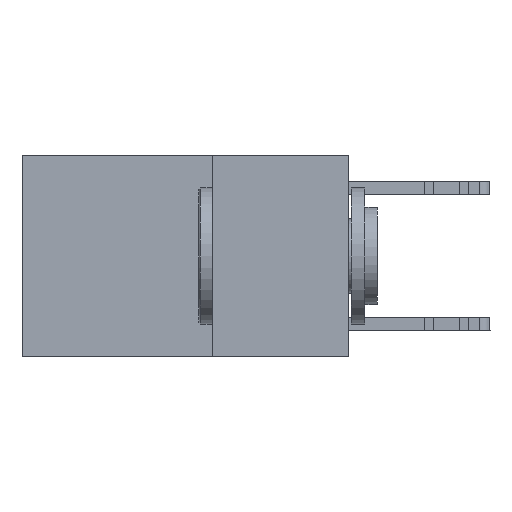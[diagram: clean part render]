
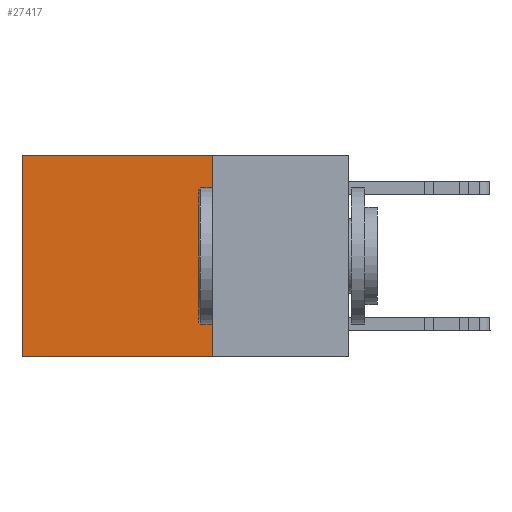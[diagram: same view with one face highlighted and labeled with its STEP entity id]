
A CAD part, left-side view. The second image highlights one B-rep face of the part: STEP entity #27417.
In plain terms, the highlighted planar face has unit normal (-1, 0, 0).
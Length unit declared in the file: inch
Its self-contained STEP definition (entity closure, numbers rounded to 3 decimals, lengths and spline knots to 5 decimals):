
#86 = CARTESIAN_POINT ( 'NONE',  ( 0.2625, 0.6, 0. ) ) ;
#890 = ORIENTED_EDGE ( 'NONE', *, *, #20399, .F. ) ;
#1608 = VECTOR ( 'NONE', #26560, 39.37008 ) ;
#1846 = LINE ( 'NONE', #5720, #1608 ) ;
#2043 = EDGE_LOOP ( 'NONE', ( #15381, #29146, #890, #13578 ) ) ;
#2847 = EDGE_CURVE ( 'NONE', #28796, #15309, #1846, .T. ) ;
#3689 = LINE ( 'NONE', #5664, #16736 ) ;
#4031 = VECTOR ( 'NONE', #9306, 39.37008 ) ;
#4497 = LINE ( 'NONE', #10166, #4031 ) ;
#4861 = VERTEX_POINT ( 'NONE', #11700 ) ;
#5664 = CARTESIAN_POINT ( 'NONE',  ( 0.2625, 0.25, -0.37 ) ) ;
#5720 = CARTESIAN_POINT ( 'NONE',  ( 0.2625, 0.25, 0. ) ) ;
#7655 = LINE ( 'NONE', #28075, #13438 ) ;
#9306 = DIRECTION ( 'NONE',  ( 0., 0., -1. ) ) ;
#10024 = CARTESIAN_POINT ( 'NONE',  ( 0.2625, 0.25, -0.37 ) ) ;
#10166 = CARTESIAN_POINT ( 'NONE',  ( 0.2625, 0.25, 0. ) ) ;
#11700 = CARTESIAN_POINT ( 'NONE',  ( 0.2625, 0.6, -0.37 ) ) ;
#13438 = VECTOR ( 'NONE', #27195, 39.37008 ) ;
#13578 = ORIENTED_EDGE ( 'NONE', *, *, #2847, .T. ) ;
#13822 = AXIS2_PLACEMENT_3D ( 'NONE', #21969, #29136, #14888 ) ;
#14818 = FACE_OUTER_BOUND ( 'NONE', #2043, .T. ) ;
#14888 = DIRECTION ( 'NONE',  ( 0., 0., -1. ) ) ;
#15309 = VERTEX_POINT ( 'NONE', #86 ) ;
#15381 = ORIENTED_EDGE ( 'NONE', *, *, #24422, .T. ) ;
#16736 = VECTOR ( 'NONE', #22611, 39.37008 ) ;
#20366 = VERTEX_POINT ( 'NONE', #10024 ) ;
#20399 = EDGE_CURVE ( 'NONE', #28796, #20366, #4497, .T. ) ;
#21969 = CARTESIAN_POINT ( 'NONE',  ( 0.2625, 0.25, 0. ) ) ;
#22611 = DIRECTION ( 'NONE',  ( 0., 1., 0. ) ) ;
#24422 = EDGE_CURVE ( 'NONE', #15309, #4861, #7655, .T. ) ;
#26560 = DIRECTION ( 'NONE',  ( 0., 1., 0. ) ) ;
#26726 = PLANE ( 'NONE',  #13822 ) ;
#27195 = DIRECTION ( 'NONE',  ( 0., 0., -1. ) ) ;
#27417 = ADVANCED_FACE ( 'NONE', ( #14818 ), #26726, .F. ) ;
#28075 = CARTESIAN_POINT ( 'NONE',  ( 0.2625, 0.6, 0. ) ) ;
#28796 = VERTEX_POINT ( 'NONE', #30113 ) ;
#29136 = DIRECTION ( 'NONE',  ( 1., 0., 0. ) ) ;
#29146 = ORIENTED_EDGE ( 'NONE', *, *, #29938, .F. ) ;
#29938 = EDGE_CURVE ( 'NONE', #20366, #4861, #3689, .T. ) ;
#30113 = CARTESIAN_POINT ( 'NONE',  ( 0.2625, 0.25, 0. ) ) ;
